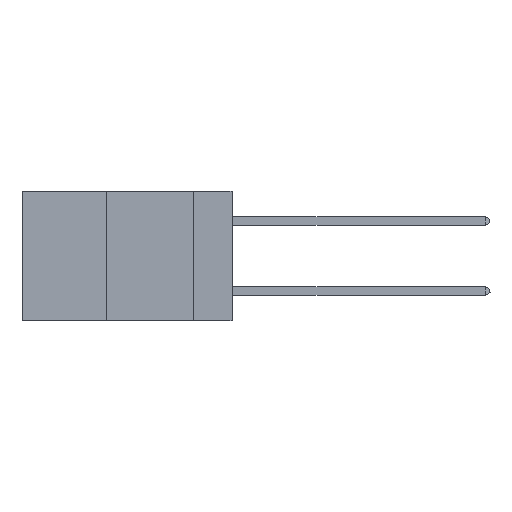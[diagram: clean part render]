
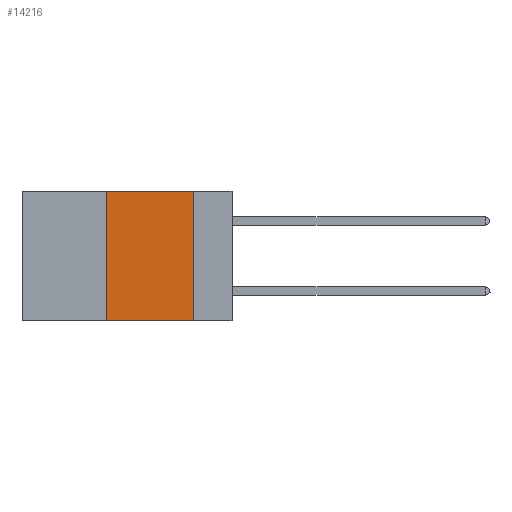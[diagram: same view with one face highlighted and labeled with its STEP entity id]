
A CAD part, left-side view. The second image highlights one B-rep face of the part: STEP entity #14216.
In plain terms, the highlighted planar face has unit normal (-1, 0, 0).
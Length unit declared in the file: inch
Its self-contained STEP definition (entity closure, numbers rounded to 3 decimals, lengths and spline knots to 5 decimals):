
#243 = FACE_OUTER_BOUND ( 'NONE', #7898, .T. ) ;
#2613 = VECTOR ( 'NONE', #29387, 39.37008 ) ;
#3655 = CARTESIAN_POINT ( 'NONE',  ( 0., 0.36, 0. ) ) ;
#3810 = DIRECTION ( 'NONE',  ( 0., -1., 0. ) ) ;
#4115 = VERTEX_POINT ( 'NONE', #18794 ) ;
#4471 = CARTESIAN_POINT ( 'NONE',  ( 0., 0.36, 0. ) ) ;
#5492 = ORIENTED_EDGE ( 'NONE', *, *, #36995, .F. ) ;
#7575 = CARTESIAN_POINT ( 'NONE',  ( 0., 0.6, -0.37 ) ) ;
#7871 = ORIENTED_EDGE ( 'NONE', *, *, #25304, .F. ) ;
#7898 = EDGE_LOOP ( 'NONE', ( #10475, #5492, #7871, #24496 ) ) ;
#9352 = CARTESIAN_POINT ( 'NONE',  ( 0., 0.6, 0. ) ) ;
#9790 = CARTESIAN_POINT ( 'NONE',  ( 0., 0.6, 0. ) ) ;
#9855 = VERTEX_POINT ( 'NONE', #4471 ) ;
#10475 = ORIENTED_EDGE ( 'NONE', *, *, #15800, .F. ) ;
#11144 = VECTOR ( 'NONE', #25965, 39.37008 ) ;
#11886 = CARTESIAN_POINT ( 'NONE',  ( 0., 0.11, 0. ) ) ;
#13266 = LINE ( 'NONE', #9790, #27635 ) ;
#14216 = ADVANCED_FACE ( 'NONE', ( #243 ), #31167, .F. ) ;
#15800 = EDGE_CURVE ( 'NONE', #20027, #27222, #28405, .T. ) ;
#15832 = LINE ( 'NONE', #3655, #16796 ) ;
#16796 = VECTOR ( 'NONE', #28104, 39.37008 ) ;
#17462 = AXIS2_PLACEMENT_3D ( 'NONE', #9352, #37309, #30891 ) ;
#18794 = CARTESIAN_POINT ( 'NONE',  ( 0., 0.36, -0.37 ) ) ;
#19819 = CARTESIAN_POINT ( 'NONE',  ( 0., 0.11, 0. ) ) ;
#20027 = VERTEX_POINT ( 'NONE', #11886 ) ;
#22697 = LINE ( 'NONE', #7575, #2613 ) ;
#24496 = ORIENTED_EDGE ( 'NONE', *, *, #29045, .T. ) ;
#25304 = EDGE_CURVE ( 'NONE', #4115, #9855, #15832, .T. ) ;
#25965 = DIRECTION ( 'NONE',  ( 0., 0., -1. ) ) ;
#27222 = VERTEX_POINT ( 'NONE', #35591 ) ;
#27635 = VECTOR ( 'NONE', #3810, 39.37008 ) ;
#28104 = DIRECTION ( 'NONE',  ( 0., 0., 1. ) ) ;
#28405 = LINE ( 'NONE', #19819, #11144 ) ;
#29045 = EDGE_CURVE ( 'NONE', #4115, #27222, #22697, .T. ) ;
#29387 = DIRECTION ( 'NONE',  ( 0., -1., 0. ) ) ;
#30891 = DIRECTION ( 'NONE',  ( 0., 0., -1. ) ) ;
#31167 = PLANE ( 'NONE',  #17462 ) ;
#35591 = CARTESIAN_POINT ( 'NONE',  ( 0., 0.11, -0.37 ) ) ;
#36995 = EDGE_CURVE ( 'NONE', #9855, #20027, #13266, .T. ) ;
#37309 = DIRECTION ( 'NONE',  ( 1., 0., 0. ) ) ;
